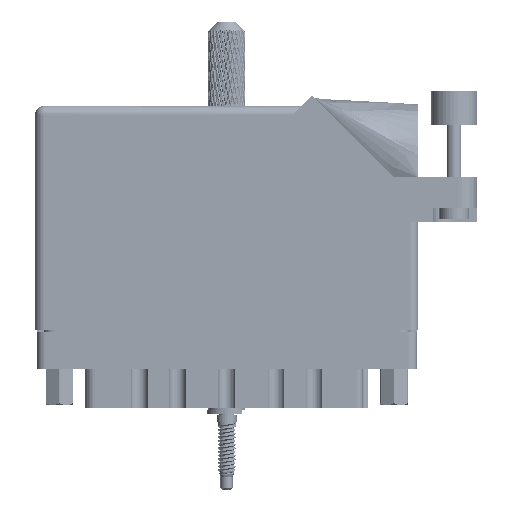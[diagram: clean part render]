
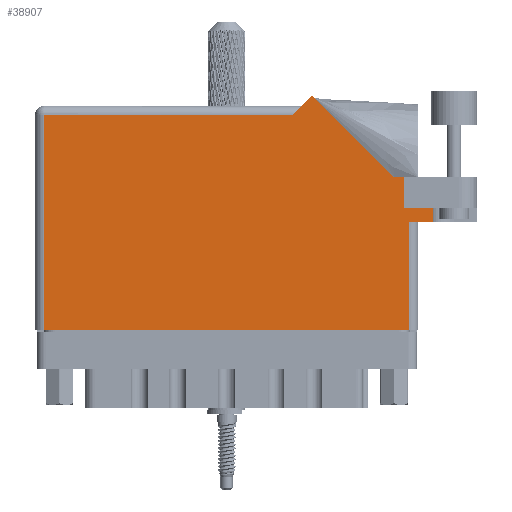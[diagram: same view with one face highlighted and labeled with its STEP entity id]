
A CAD part, front view. The second image highlights one B-rep face of the part: STEP entity #38907.
In plain terms, the highlighted face is planar.
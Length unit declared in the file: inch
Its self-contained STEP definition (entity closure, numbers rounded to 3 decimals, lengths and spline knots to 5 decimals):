
#6266 = DIRECTION ( 'NONE',  ( 1., 0., 0. ) ) ;
#7192 = VECTOR ( 'NONE', #51719, 39.37008 ) ;
#8309 = CARTESIAN_POINT ( 'NONE',  ( 0., 0., 0. ) ) ;
#8567 = VERTEX_POINT ( 'NONE', #100510 ) ;
#8694 = CARTESIAN_POINT ( 'NONE',  ( 0.062, 0., 0. ) ) ;
#9891 = ORIENTED_EDGE ( 'NONE', *, *, #35644, .F. ) ;
#10271 = LINE ( 'NONE', #57277, #24173 ) ;
#12374 = LINE ( 'NONE', #8694, #114721 ) ;
#14200 = CARTESIAN_POINT ( 'NONE',  ( 2.7135, 1.16177, 0. ) ) ;
#16950 = ORIENTED_EDGE ( 'NONE', *, *, #108194, .T. ) ;
#17153 = VECTOR ( 'NONE', #66143, 39.37008 ) ;
#18164 = DIRECTION ( 'NONE',  ( 0., -1., 0. ) ) ;
#19339 = VECTOR ( 'NONE', #84429, 39.37008 ) ;
#20082 = CARTESIAN_POINT ( 'NONE',  ( 0., 1.468, 0. ) ) ;
#24173 = VECTOR ( 'NONE', #87727, 39.37008 ) ;
#25462 = CARTESIAN_POINT ( 'NONE',  ( 2.7135, 0.737, 0. ) ) ;
#25706 = VERTEX_POINT ( 'NONE', #84958 ) ;
#25877 = EDGE_CURVE ( 'NONE', #25706, #116613, #55293, .T. ) ;
#27588 = VERTEX_POINT ( 'NONE', #91005 ) ;
#28828 = PLANE ( 'NONE',  #103229 ) ;
#29023 = EDGE_CURVE ( 'NONE', #8567, #40592, #40769, .T. ) ;
#30429 = VECTOR ( 'NONE', #48470, 39.37008 ) ;
#30471 = CARTESIAN_POINT ( 'NONE',  ( 1.88971, 1.60071, 0. ) ) ;
#35644 = EDGE_CURVE ( 'NONE', #40592, #100579, #83825, .T. ) ;
#35917 = CARTESIAN_POINT ( 'NONE',  ( 2.44642, 1.044, 0. ) ) ;
#36273 = CARTESIAN_POINT ( 'NONE',  ( 1.819, 1.53, 0. ) ) ;
#37749 = LINE ( 'NONE', #64538, #109247 ) ;
#38907 = ADVANCED_FACE ( 'NONE', ( #94225 ), #28828, .F. ) ;
#39379 = VERTEX_POINT ( 'NONE', #111885 ) ;
#40592 = VERTEX_POINT ( 'NONE', #117528 ) ;
#40769 = LINE ( 'NONE', #86062, #116801 ) ;
#40905 = EDGE_CURVE ( 'NONE', #63967, #100579, #37749, .T. ) ;
#43104 = ORIENTED_EDGE ( 'NONE', *, *, #29023, .F. ) ;
#43481 = VECTOR ( 'NONE', #84442, 39.37008 ) ;
#44475 = EDGE_CURVE ( 'NONE', #116613, #64509, #110173, .T. ) ;
#44945 = CARTESIAN_POINT ( 'NONE',  ( 2.55, 0.737, 0. ) ) ;
#47695 = DIRECTION ( 'NONE',  ( 1., 0., 0. ) ) ;
#48470 = DIRECTION ( 'NONE',  ( -0.707, 0.707, 0. ) ) ;
#48967 = ORIENTED_EDGE ( 'NONE', *, *, #98347, .T. ) ;
#51719 = DIRECTION ( 'NONE',  ( -1., 0., 0. ) ) ;
#55156 = VERTEX_POINT ( 'NONE', #106049 ) ;
#55293 = LINE ( 'NONE', #35917, #30429 ) ;
#57277 = CARTESIAN_POINT ( 'NONE',  ( 2.512, 0.831, 0. ) ) ;
#61907 = ORIENTED_EDGE ( 'NONE', *, *, #104404, .T. ) ;
#63967 = VERTEX_POINT ( 'NONE', #95996 ) ;
#64509 = VERTEX_POINT ( 'NONE', #98917 ) ;
#64538 = CARTESIAN_POINT ( 'NONE',  ( 2.612, 0.737, 0. ) ) ;
#65314 = EDGE_LOOP ( 'NONE', ( #61907, #48967, #69868, #9891, #43104, #114622, #84833, #79956, #69613, #117420, #16950 ) ) ;
#66143 = DIRECTION ( 'NONE',  ( -0.707, -0.707, 0. ) ) ;
#69613 = ORIENTED_EDGE ( 'NONE', *, *, #44475, .T. ) ;
#69868 = ORIENTED_EDGE ( 'NONE', *, *, #40905, .T. ) ;
#72025 = LINE ( 'NONE', #44945, #19339 ) ;
#73735 = LINE ( 'NONE', #20082, #7192 ) ;
#74567 = EDGE_CURVE ( 'NONE', #103064, #25706, #125185, .T. ) ;
#79956 = ORIENTED_EDGE ( 'NONE', *, *, #25877, .T. ) ;
#83234 = EDGE_CURVE ( 'NONE', #64509, #55156, #73735, .T. ) ;
#83510 = EDGE_CURVE ( 'NONE', #8567, #103064, #10271, .T. ) ;
#83825 = LINE ( 'NONE', #14200, #43481 ) ;
#84245 = VECTOR ( 'NONE', #47695, 39.37008 ) ;
#84429 = DIRECTION ( 'NONE',  ( 0., 1., 0. ) ) ;
#84442 = DIRECTION ( 'NONE',  ( 0., -1., 0. ) ) ;
#84833 = ORIENTED_EDGE ( 'NONE', *, *, #74567, .T. ) ;
#84958 = CARTESIAN_POINT ( 'NONE',  ( 2.44642, 1.044, 0. ) ) ;
#86062 = CARTESIAN_POINT ( 'NONE',  ( 2.512, 0.831, 0. ) ) ;
#87727 = DIRECTION ( 'NONE',  ( 0., 1., 0. ) ) ;
#91005 = CARTESIAN_POINT ( 'NONE',  ( 0.062, 0., 0. ) ) ;
#94225 = FACE_OUTER_BOUND ( 'NONE', #65314, .T. ) ;
#95996 = CARTESIAN_POINT ( 'NONE',  ( 2.55, 0.737, 0. ) ) ;
#98347 = EDGE_CURVE ( 'NONE', #39379, #63967, #72025, .T. ) ;
#98917 = CARTESIAN_POINT ( 'NONE',  ( 1.757, 1.468, 0. ) ) ;
#100510 = CARTESIAN_POINT ( 'NONE',  ( 2.512, 0.831, 0. ) ) ;
#100579 = VERTEX_POINT ( 'NONE', #25462 ) ;
#103064 = VERTEX_POINT ( 'NONE', #121187 ) ;
#103229 = AXIS2_PLACEMENT_3D ( 'NONE', #108175, #118155, #128113 ) ;
#104017 = DIRECTION ( 'NONE',  ( 1., 0., 0. ) ) ;
#104404 = EDGE_CURVE ( 'NONE', #27588, #39379, #119889, .T. ) ;
#105002 = VECTOR ( 'NONE', #105965, 39.37008 ) ;
#105965 = DIRECTION ( 'NONE',  ( -1., 0., 0. ) ) ;
#106049 = CARTESIAN_POINT ( 'NONE',  ( 0.062, 1.468, 0. ) ) ;
#108175 = CARTESIAN_POINT ( 'NONE',  ( 0., 1.53, 0. ) ) ;
#108194 = EDGE_CURVE ( 'NONE', #55156, #27588, #12374, .T. ) ;
#109247 = VECTOR ( 'NONE', #104017, 39.37008 ) ;
#110173 = LINE ( 'NONE', #36273, #17153 ) ;
#111885 = CARTESIAN_POINT ( 'NONE',  ( 2.55, 0., 0. ) ) ;
#114622 = ORIENTED_EDGE ( 'NONE', *, *, #83510, .T. ) ;
#114721 = VECTOR ( 'NONE', #18164, 39.37008 ) ;
#116613 = VERTEX_POINT ( 'NONE', #30471 ) ;
#116801 = VECTOR ( 'NONE', #6266, 39.37008 ) ;
#117420 = ORIENTED_EDGE ( 'NONE', *, *, #83234, .T. ) ;
#117528 = CARTESIAN_POINT ( 'NONE',  ( 2.7135, 0.831, 0. ) ) ;
#118155 = DIRECTION ( 'NONE',  ( 0., 0., -1. ) ) ;
#119889 = LINE ( 'NONE', #8309, #84245 ) ;
#121187 = CARTESIAN_POINT ( 'NONE',  ( 2.512, 1.044, 0. ) ) ;
#125185 = LINE ( 'NONE', #125487, #105002 ) ;
#125487 = CARTESIAN_POINT ( 'NONE',  ( 3.012, 1.044, 0. ) ) ;
#128113 = DIRECTION ( 'NONE',  ( -1., 0., 0. ) ) ;
